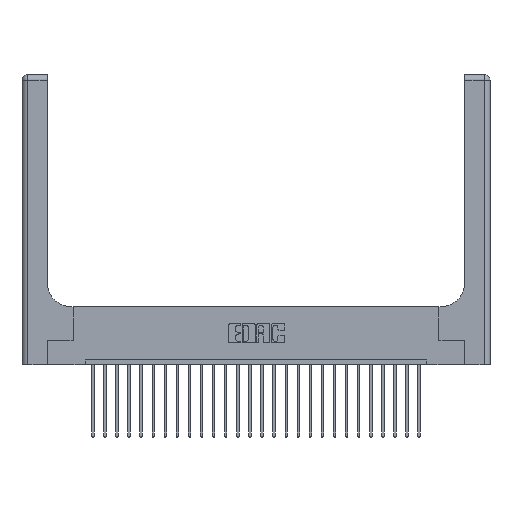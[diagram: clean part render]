
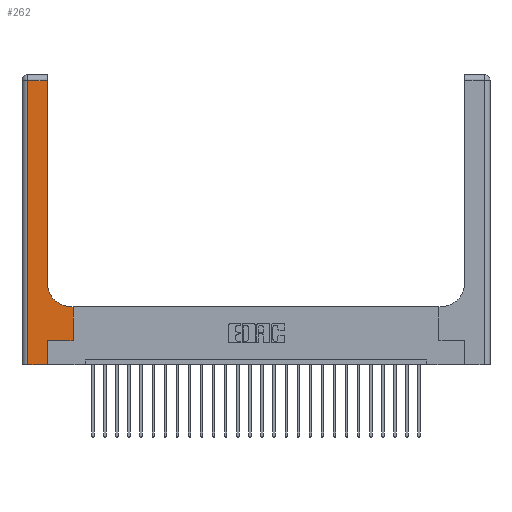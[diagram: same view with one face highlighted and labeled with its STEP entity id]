
A CAD part, top view. The second image highlights one B-rep face of the part: STEP entity #262.
In plain terms, the highlighted planar face has unit normal (0, 0, 1).
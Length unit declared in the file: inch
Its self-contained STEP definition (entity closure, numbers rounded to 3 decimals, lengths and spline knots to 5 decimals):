
#129 = LINE ( 'NONE', #6184, #5443 ) ;
#262 = ADVANCED_FACE ( 'NONE', ( #2915 ), #2505, .F. ) ;
#265 = VECTOR ( 'NONE', #1956, 39.37008 ) ;
#726 = DIRECTION ( 'NONE',  ( 0., -1., 0. ) ) ;
#1123 = DIRECTION ( 'NONE',  ( 0., 0., -1. ) ) ;
#1517 = VERTEX_POINT ( 'NONE', #14654 ) ;
#1956 = DIRECTION ( 'NONE',  ( 1., 0., 0. ) ) ;
#2366 = CARTESIAN_POINT ( 'NONE',  ( 0.06, 3., 0.37 ) ) ;
#2425 = DIRECTION ( 'NONE',  ( 0., 1., 0. ) ) ;
#2505 = PLANE ( 'NONE',  #6850 ) ;
#2862 = VERTEX_POINT ( 'NONE', #6551 ) ;
#2915 = FACE_OUTER_BOUND ( 'NONE', #20088, .T. ) ;
#2919 = ORIENTED_EDGE ( 'NONE', *, *, #20330, .T. ) ;
#3235 = CARTESIAN_POINT ( 'NONE',  ( 0., 2.94, 0.37 ) ) ;
#3260 = VERTEX_POINT ( 'NONE', #6030 ) ;
#3545 = ORIENTED_EDGE ( 'NONE', *, *, #24059, .T. ) ;
#3979 = VERTEX_POINT ( 'NONE', #6489 ) ;
#4176 = EDGE_CURVE ( 'NONE', #1517, #3979, #10395, .T. ) ;
#4375 = DIRECTION ( 'NONE',  ( 0., 1., 0. ) ) ;
#4582 = LINE ( 'NONE', #6230, #24066 ) ;
#4622 = ORIENTED_EDGE ( 'NONE', *, *, #12926, .T. ) ;
#4645 = EDGE_CURVE ( 'NONE', #21814, #2862, #17485, .T. ) ;
#5072 = DIRECTION ( 'NONE',  ( -1., 0., 0. ) ) ;
#5406 = VECTOR ( 'NONE', #7053, 39.37008 ) ;
#5425 = VECTOR ( 'NONE', #11647, 39.37008 ) ;
#5443 = VECTOR ( 'NONE', #13614, 39.37008 ) ;
#5536 = ORIENTED_EDGE ( 'NONE', *, *, #23795, .T. ) ;
#5687 = ORIENTED_EDGE ( 'NONE', *, *, #9469, .T. ) ;
#6030 = CARTESIAN_POINT ( 'NONE',  ( 0.06, 2.94, 0.37 ) ) ;
#6184 = CARTESIAN_POINT ( 'NONE',  ( 0.26, 3., 0.37 ) ) ;
#6230 = CARTESIAN_POINT ( 'NONE',  ( 0.265, 0., 0.37 ) ) ;
#6489 = CARTESIAN_POINT ( 'NONE',  ( 0.265, 0., 0.37 ) ) ;
#6551 = CARTESIAN_POINT ( 'NONE',  ( 0.26, 0.85, 0.37 ) ) ;
#6850 = AXIS2_PLACEMENT_3D ( 'NONE', #21187, #10264, #16059 ) ;
#7053 = DIRECTION ( 'NONE',  ( 1., 0., 0. ) ) ;
#7663 = CARTESIAN_POINT ( 'NONE',  ( 0.528, 0.25, 0.37 ) ) ;
#7970 = VERTEX_POINT ( 'NONE', #21099 ) ;
#9002 = VERTEX_POINT ( 'NONE', #16208 ) ;
#9469 = EDGE_CURVE ( 'NONE', #17654, #7970, #11196, .T. ) ;
#10115 = VERTEX_POINT ( 'NONE', #12868 ) ;
#10156 = ORIENTED_EDGE ( 'NONE', *, *, #4645, .T. ) ;
#10264 = DIRECTION ( 'NONE',  ( 0., 0., -1. ) ) ;
#10395 = LINE ( 'NONE', #14598, #5406 ) ;
#10725 = AXIS2_PLACEMENT_3D ( 'NONE', #20047, #1123, #14333 ) ;
#10792 = ORIENTED_EDGE ( 'NONE', *, *, #22644, .T. ) ;
#11196 = LINE ( 'NONE', #15866, #13279 ) ;
#11454 = EDGE_CURVE ( 'NONE', #9002, #3260, #14329, .T. ) ;
#11647 = DIRECTION ( 'NONE',  ( -1., 0., 0. ) ) ;
#12868 = CARTESIAN_POINT ( 'NONE',  ( 0.265, 0.25, 0.37 ) ) ;
#12926 = EDGE_CURVE ( 'NONE', #3260, #1517, #17850, .T. ) ;
#13279 = VECTOR ( 'NONE', #4375, 39.37008 ) ;
#13614 = DIRECTION ( 'NONE',  ( 0., 1., 0. ) ) ;
#14329 = LINE ( 'NONE', #3235, #20864 ) ;
#14333 = DIRECTION ( 'NONE',  ( 1., 0., 0. ) ) ;
#14598 = CARTESIAN_POINT ( 'NONE',  ( 0., 0., 0.37 ) ) ;
#14654 = CARTESIAN_POINT ( 'NONE',  ( 0.06, 0., 0.37 ) ) ;
#15287 = CARTESIAN_POINT ( 'NONE',  ( 0.265, 0.25, 0.37 ) ) ;
#15866 = CARTESIAN_POINT ( 'NONE',  ( 0.528, 0.25, 0.37 ) ) ;
#16059 = DIRECTION ( 'NONE',  ( -1., 0., 0. ) ) ;
#16208 = CARTESIAN_POINT ( 'NONE',  ( 0.26, 2.94, 0.37 ) ) ;
#17485 = CIRCLE ( 'NONE', #10725, 0.25 ) ;
#17654 = VERTEX_POINT ( 'NONE', #7663 ) ;
#17826 = LINE ( 'NONE', #22920, #5425 ) ;
#17850 = LINE ( 'NONE', #2366, #20813 ) ;
#18038 = ORIENTED_EDGE ( 'NONE', *, *, #11454, .T. ) ;
#18686 = CARTESIAN_POINT ( 'NONE',  ( 0.51, 0.6, 0.37 ) ) ;
#20047 = CARTESIAN_POINT ( 'NONE',  ( 0.51, 0.85, 0.37 ) ) ;
#20088 = EDGE_LOOP ( 'NONE', ( #5536, #18038, #4622, #22329, #10792, #2919, #5687, #3545, #10156 ) ) ;
#20330 = EDGE_CURVE ( 'NONE', #10115, #17654, #20633, .T. ) ;
#20633 = LINE ( 'NONE', #15287, #265 ) ;
#20813 = VECTOR ( 'NONE', #726, 39.37008 ) ;
#20864 = VECTOR ( 'NONE', #5072, 39.37008 ) ;
#21099 = CARTESIAN_POINT ( 'NONE',  ( 0.528, 0.6, 0.37 ) ) ;
#21187 = CARTESIAN_POINT ( 'NONE',  ( 0., 3., 0.37 ) ) ;
#21814 = VERTEX_POINT ( 'NONE', #18686 ) ;
#22329 = ORIENTED_EDGE ( 'NONE', *, *, #4176, .T. ) ;
#22644 = EDGE_CURVE ( 'NONE', #3979, #10115, #4582, .T. ) ;
#22920 = CARTESIAN_POINT ( 'NONE',  ( 0.26, 0.6, 0.37 ) ) ;
#23795 = EDGE_CURVE ( 'NONE', #2862, #9002, #129, .T. ) ;
#24059 = EDGE_CURVE ( 'NONE', #7970, #21814, #17826, .T. ) ;
#24066 = VECTOR ( 'NONE', #2425, 39.37008 ) ;
